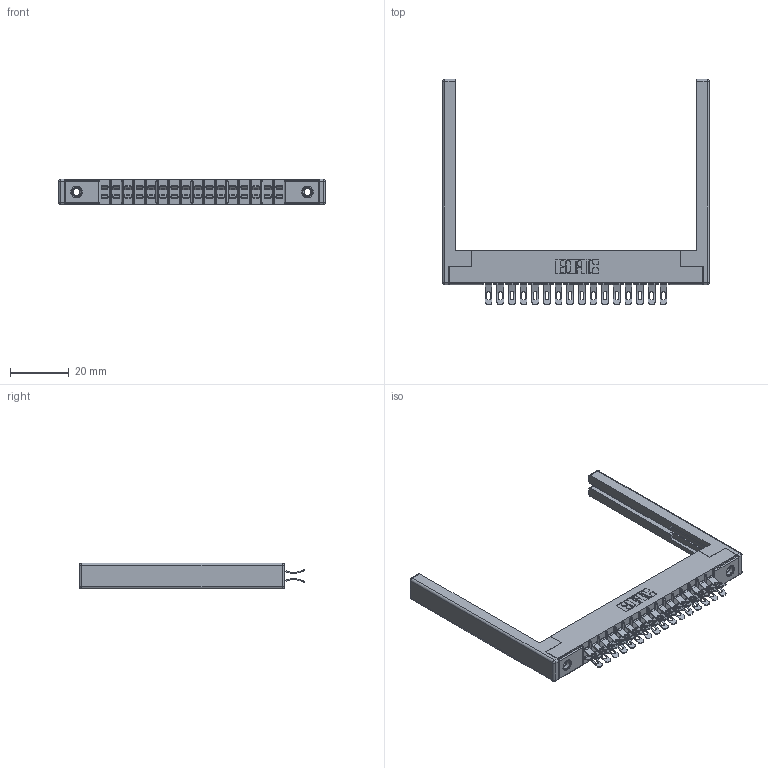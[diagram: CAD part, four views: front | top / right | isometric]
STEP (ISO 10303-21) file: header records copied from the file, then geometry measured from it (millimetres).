
FILE_DESCRIPTION (( 'STEP AP203' ), '1' );
FILE_NAME ('315-032-555-268.STEP', '2019-09-10T15:43:51', ( '' ), ( '' ), 'SwSTEP 2.0', 'SolidWorks 2016', '' );
FILE_SCHEMA (( 'CONFIG_CONTROL_DESIGN' ));
Length unit declared in the file: inch
Products named in the file (5): 305 Part_.156 Dia; 345-250-001_345-250-001-102; 307-220-068; 315-032-555-268; 305-290-001_555
Assembly tree (37 placements, depth 2):
  315-032-555-268
    305 Part_.156 Dia
    305-290-001_555  x32
    345-250-001_345-250-001-102  x2
    307-220-068  x2
Bounding box: 90.83 x 76.71 x 8.71 mm (x, y, z)
Volume: 10377.6 mm3; surface area: 15170.5 mm2
Topology: 37 solids, 37 shells, 2382 faces, 7026 edges, 4576 vertices
Faces by surface type: plane 1180, cylinder 1114, sphere 72, cone 12, torus 4
Entity records: 23872 total; most frequent: CARTESIAN_POINT 3941, ORIENTED_EDGE 3890, DIRECTION 3847, EDGE_CURVE 1945, LINE 1515, VECTOR 1515, VERTEX_POINT 1244, AXIS2_PLACEMENT_3D 1166
